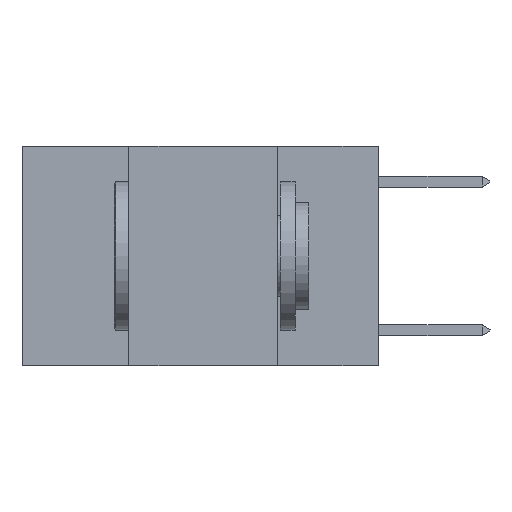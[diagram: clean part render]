
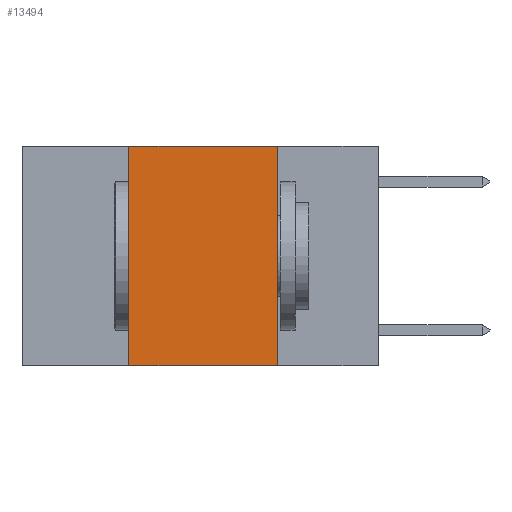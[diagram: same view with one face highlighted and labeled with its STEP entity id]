
A CAD part, left-side view. The second image highlights one B-rep face of the part: STEP entity #13494.
In plain terms, the highlighted planar face has unit normal (-1, 0, 0).
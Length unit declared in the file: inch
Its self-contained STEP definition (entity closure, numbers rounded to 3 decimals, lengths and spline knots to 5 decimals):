
#111 = ORIENTED_EDGE ( 'NONE', *, *, #18501, .F. ) ;
#726 = CARTESIAN_POINT ( 'NONE',  ( 0., 0.6, 0. ) ) ;
#1398 = CARTESIAN_POINT ( 'NONE',  ( 0., 0.42, 0. ) ) ;
#2002 = LINE ( 'NONE', #9103, #13724 ) ;
#2310 = DIRECTION ( 'NONE',  ( 0., 0., -1. ) ) ;
#3688 = EDGE_LOOP ( 'NONE', ( #5616, #5063, #111, #10747 ) ) ;
#4007 = CARTESIAN_POINT ( 'NONE',  ( 0., 0.17, 0. ) ) ;
#5063 = ORIENTED_EDGE ( 'NONE', *, *, #9672, .F. ) ;
#5143 = CARTESIAN_POINT ( 'NONE',  ( 0., 0.17, 0. ) ) ;
#5616 = ORIENTED_EDGE ( 'NONE', *, *, #15585, .F. ) ;
#6836 = DIRECTION ( 'NONE',  ( 0., -1., 0. ) ) ;
#6975 = PLANE ( 'NONE',  #7596 ) ;
#7065 = CARTESIAN_POINT ( 'NONE',  ( 0., 0.42, 0. ) ) ;
#7596 = AXIS2_PLACEMENT_3D ( 'NONE', #726, #11521, #2310 ) ;
#7709 = VERTEX_POINT ( 'NONE', #14277 ) ;
#7909 = LINE ( 'NONE', #7065, #11442 ) ;
#8647 = DIRECTION ( 'NONE',  ( 0., 0., -1. ) ) ;
#9103 = CARTESIAN_POINT ( 'NONE',  ( 0., 0.6, 0. ) ) ;
#9550 = VERTEX_POINT ( 'NONE', #5143 ) ;
#9672 = EDGE_CURVE ( 'NONE', #17405, #9550, #2002, .T. ) ;
#10437 = FACE_OUTER_BOUND ( 'NONE', #3688, .T. ) ;
#10747 = ORIENTED_EDGE ( 'NONE', *, *, #13439, .T. ) ;
#11442 = VECTOR ( 'NONE', #17449, 39.37008 ) ;
#11521 = DIRECTION ( 'NONE',  ( 1., 0., 0. ) ) ;
#12722 = LINE ( 'NONE', #4007, #19136 ) ;
#13439 = EDGE_CURVE ( 'NONE', #14869, #7709, #15838, .T. ) ;
#13494 = ADVANCED_FACE ( 'NONE', ( #10437 ), #6975, .F. ) ;
#13724 = VECTOR ( 'NONE', #14107, 39.37008 ) ;
#14107 = DIRECTION ( 'NONE',  ( 0., -1., 0. ) ) ;
#14277 = CARTESIAN_POINT ( 'NONE',  ( 0., 0.17, -0.37 ) ) ;
#14869 = VERTEX_POINT ( 'NONE', #18943 ) ;
#15362 = VECTOR ( 'NONE', #6836, 39.37008 ) ;
#15585 = EDGE_CURVE ( 'NONE', #9550, #7709, #12722, .T. ) ;
#15838 = LINE ( 'NONE', #18691, #15362 ) ;
#17405 = VERTEX_POINT ( 'NONE', #1398 ) ;
#17449 = DIRECTION ( 'NONE',  ( 0., 0., 1. ) ) ;
#18501 = EDGE_CURVE ( 'NONE', #14869, #17405, #7909, .T. ) ;
#18691 = CARTESIAN_POINT ( 'NONE',  ( 0., 0.6, -0.37 ) ) ;
#18943 = CARTESIAN_POINT ( 'NONE',  ( 0., 0.42, -0.37 ) ) ;
#19136 = VECTOR ( 'NONE', #8647, 39.37008 ) ;
